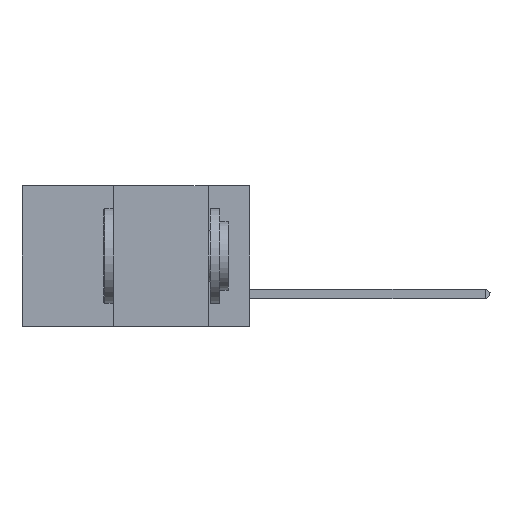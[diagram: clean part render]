
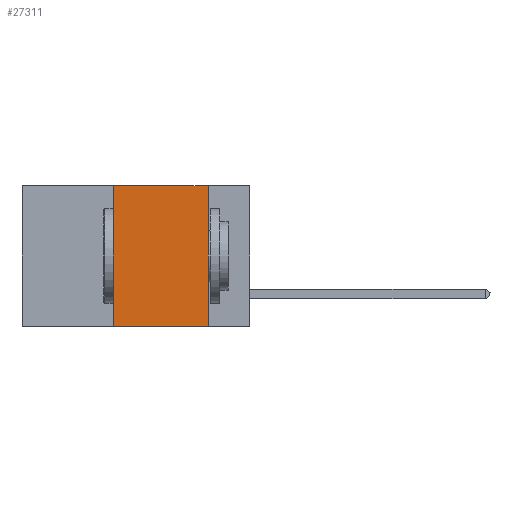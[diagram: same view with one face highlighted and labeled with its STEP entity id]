
A CAD part, left-side view. The second image highlights one B-rep face of the part: STEP entity #27311.
In plain terms, the highlighted planar face has unit normal (-1, 0, 0).
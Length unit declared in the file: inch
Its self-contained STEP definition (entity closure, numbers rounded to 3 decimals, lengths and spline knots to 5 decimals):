
#1484 = CARTESIAN_POINT ( 'NONE',  ( 0., 0.36, -0.37 ) ) ;
#1699 = VERTEX_POINT ( 'NONE', #1484 ) ;
#2969 = CARTESIAN_POINT ( 'NONE',  ( 0., 0.11, 0. ) ) ;
#3096 = DIRECTION ( 'NONE',  ( 0., 0., -1. ) ) ;
#3186 = VECTOR ( 'NONE', #7290, 39.37008 ) ;
#4525 = ORIENTED_EDGE ( 'NONE', *, *, #33696, .F. ) ;
#5755 = DIRECTION ( 'NONE',  ( 1., 0., 0. ) ) ;
#6622 = EDGE_LOOP ( 'NONE', ( #17151, #4525, #34908, #19654 ) ) ;
#6664 = VERTEX_POINT ( 'NONE', #2969 ) ;
#7290 = DIRECTION ( 'NONE',  ( 0., -1., 0. ) ) ;
#7451 = LINE ( 'NONE', #22672, #38739 ) ;
#10431 = LINE ( 'NONE', #21377, #36505 ) ;
#10543 = CARTESIAN_POINT ( 'NONE',  ( 0., 0.11, -0.37 ) ) ;
#11344 = AXIS2_PLACEMENT_3D ( 'NONE', #29392, #5755, #3096 ) ;
#11575 = VERTEX_POINT ( 'NONE', #10543 ) ;
#12512 = FACE_OUTER_BOUND ( 'NONE', #6622, .T. ) ;
#13196 = CARTESIAN_POINT ( 'NONE',  ( 0., 0.6, -0.37 ) ) ;
#16553 = EDGE_CURVE ( 'NONE', #1699, #11575, #22984, .T. ) ;
#17151 = ORIENTED_EDGE ( 'NONE', *, *, #19688, .F. ) ;
#19654 = ORIENTED_EDGE ( 'NONE', *, *, #16553, .T. ) ;
#19688 = EDGE_CURVE ( 'NONE', #6664, #11575, #7451, .T. ) ;
#21377 = CARTESIAN_POINT ( 'NONE',  ( 0., 0.36, 0. ) ) ;
#22582 = DIRECTION ( 'NONE',  ( 0., -1., 0. ) ) ;
#22672 = CARTESIAN_POINT ( 'NONE',  ( 0., 0.11, 0. ) ) ;
#22984 = LINE ( 'NONE', #13196, #29083 ) ;
#24439 = DIRECTION ( 'NONE',  ( 0., 0., 1. ) ) ;
#27311 = ADVANCED_FACE ( 'NONE', ( #12512 ), #29800, .F. ) ;
#28757 = EDGE_CURVE ( 'NONE', #1699, #34117, #10431, .T. ) ;
#28977 = DIRECTION ( 'NONE',  ( 0., 0., -1. ) ) ;
#29083 = VECTOR ( 'NONE', #22582, 39.37008 ) ;
#29392 = CARTESIAN_POINT ( 'NONE',  ( 0., 0.6, 0. ) ) ;
#29800 = PLANE ( 'NONE',  #11344 ) ;
#30426 = CARTESIAN_POINT ( 'NONE',  ( 0., 0.36, 0. ) ) ;
#33696 = EDGE_CURVE ( 'NONE', #34117, #6664, #39191, .T. ) ;
#34117 = VERTEX_POINT ( 'NONE', #30426 ) ;
#34428 = CARTESIAN_POINT ( 'NONE',  ( 0., 0.6, 0. ) ) ;
#34908 = ORIENTED_EDGE ( 'NONE', *, *, #28757, .F. ) ;
#36505 = VECTOR ( 'NONE', #24439, 39.37008 ) ;
#38739 = VECTOR ( 'NONE', #28977, 39.37008 ) ;
#39191 = LINE ( 'NONE', #34428, #3186 ) ;
